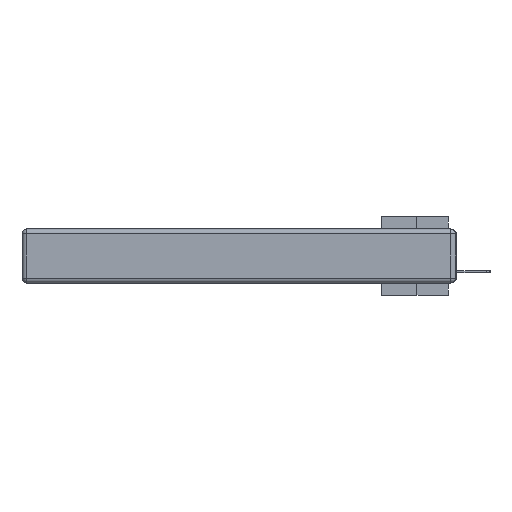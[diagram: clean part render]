
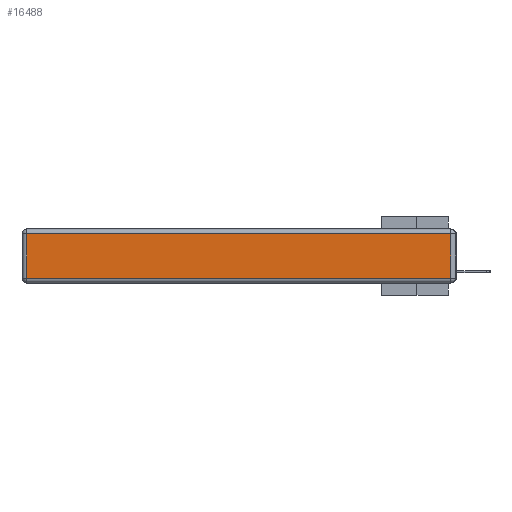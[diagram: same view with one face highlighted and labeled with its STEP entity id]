
A CAD part, left-side view. The second image highlights one B-rep face of the part: STEP entity #16488.
In plain terms, the highlighted planar face has unit normal (-1, 0, 0).
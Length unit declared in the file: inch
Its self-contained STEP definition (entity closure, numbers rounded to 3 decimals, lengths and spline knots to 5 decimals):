
#391 = VERTEX_POINT ( 'NONE', #1556 ) ;
#1556 = CARTESIAN_POINT ( 'NONE',  ( 0., 2.72, -0.313 ) ) ;
#2003 = ORIENTED_EDGE ( 'NONE', *, *, #17177, .T. ) ;
#2386 = VECTOR ( 'NONE', #13860, 39.37008 ) ;
#2798 = CARTESIAN_POINT ( 'NONE',  ( 0., 2.72, -0.03 ) ) ;
#4984 = ORIENTED_EDGE ( 'NONE', *, *, #8850, .T. ) ;
#5553 = VECTOR ( 'NONE', #24039, 39.37008 ) ;
#5783 = CARTESIAN_POINT ( 'NONE',  ( 0., 2.72, -0.343 ) ) ;
#6157 = VERTEX_POINT ( 'NONE', #17277 ) ;
#6392 = CARTESIAN_POINT ( 'NONE',  ( 0., 0.03, -0.313 ) ) ;
#7758 = VECTOR ( 'NONE', #19262, 39.37008 ) ;
#7772 = EDGE_LOOP ( 'NONE', ( #25253, #2003, #4984, #14493 ) ) ;
#7919 = LINE ( 'NONE', #18432, #2386 ) ;
#7956 = CARTESIAN_POINT ( 'NONE',  ( 0., 2.75, -0.03 ) ) ;
#8850 = EDGE_CURVE ( 'NONE', #6157, #18216, #23753, .T. ) ;
#9634 = FACE_OUTER_BOUND ( 'NONE', #7772, .T. ) ;
#9824 = DIRECTION ( 'NONE',  ( 0., 0., 1. ) ) ;
#10096 = CARTESIAN_POINT ( 'NONE',  ( 0., 0.03, -0.343 ) ) ;
#12448 = LINE ( 'NONE', #5783, #5553 ) ;
#13860 = DIRECTION ( 'NONE',  ( 0., -1., 0. ) ) ;
#14493 = ORIENTED_EDGE ( 'NONE', *, *, #17248, .T. ) ;
#16488 = ADVANCED_FACE ( 'NONE', ( #9634 ), #23310, .T. ) ;
#17177 = EDGE_CURVE ( 'NONE', #28858, #6157, #19942, .T. ) ;
#17248 = EDGE_CURVE ( 'NONE', #18216, #391, #12448, .T. ) ;
#17277 = CARTESIAN_POINT ( 'NONE',  ( 0., 0.03, -0.03 ) ) ;
#17779 = VECTOR ( 'NONE', #21650, 39.37008 ) ;
#18216 = VERTEX_POINT ( 'NONE', #2798 ) ;
#18432 = CARTESIAN_POINT ( 'NONE',  ( 0., 0., -0.313 ) ) ;
#19262 = DIRECTION ( 'NONE',  ( 0., 0., 1. ) ) ;
#19942 = LINE ( 'NONE', #10096, #7758 ) ;
#20105 = EDGE_CURVE ( 'NONE', #391, #28858, #7919, .T. ) ;
#21195 = CARTESIAN_POINT ( 'NONE',  ( 0., 0., -0.343 ) ) ;
#21650 = DIRECTION ( 'NONE',  ( 0., 1., 0. ) ) ;
#22281 = AXIS2_PLACEMENT_3D ( 'NONE', #21195, #23410, #9824 ) ;
#23310 = PLANE ( 'NONE',  #22281 ) ;
#23410 = DIRECTION ( 'NONE',  ( -1., 0., 0. ) ) ;
#23753 = LINE ( 'NONE', #7956, #17779 ) ;
#24039 = DIRECTION ( 'NONE',  ( 0., 0., -1. ) ) ;
#25253 = ORIENTED_EDGE ( 'NONE', *, *, #20105, .T. ) ;
#28858 = VERTEX_POINT ( 'NONE', #6392 ) ;
